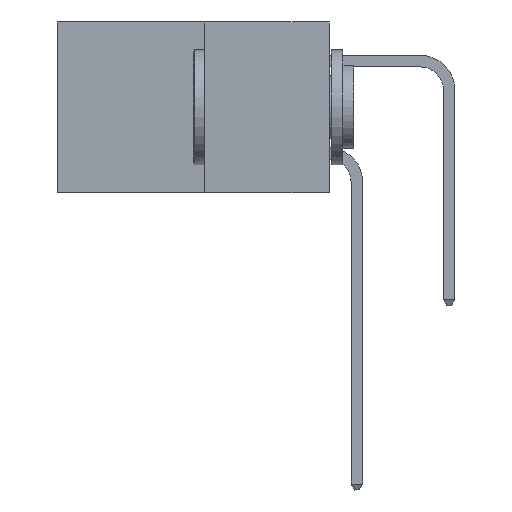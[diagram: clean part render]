
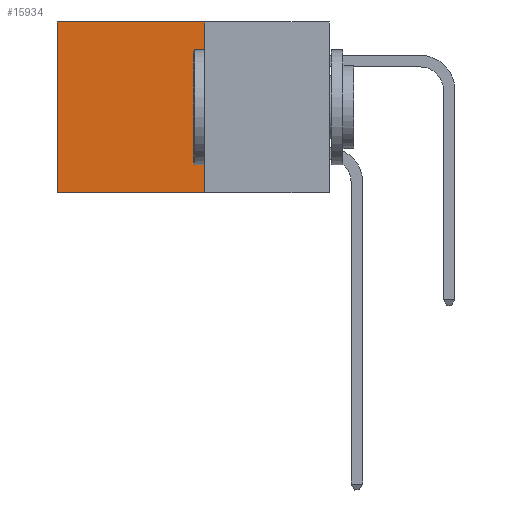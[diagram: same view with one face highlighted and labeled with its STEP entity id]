
A CAD part, left-side view. The second image highlights one B-rep face of the part: STEP entity #15934.
In plain terms, the highlighted planar face has unit normal (-1, 0, 0).
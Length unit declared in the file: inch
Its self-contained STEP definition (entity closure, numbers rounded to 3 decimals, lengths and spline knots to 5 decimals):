
#516 = VECTOR ( 'NONE', #14558, 39.37008 ) ;
#780 = VERTEX_POINT ( 'NONE', #2184 ) ;
#958 = ORIENTED_EDGE ( 'NONE', *, *, #1210, .T. ) ;
#1210 = EDGE_CURVE ( 'NONE', #10271, #9651, #15491, .T. ) ;
#2184 = CARTESIAN_POINT ( 'NONE',  ( 0.277, 0.27, 0. ) ) ;
#3373 = EDGE_CURVE ( 'NONE', #10258, #9651, #12716, .T. ) ;
#3897 = CARTESIAN_POINT ( 'NONE',  ( 0.277, 0.27, 0. ) ) ;
#4128 = CARTESIAN_POINT ( 'NONE',  ( 0.277, 0.59, -0.37 ) ) ;
#5080 = DIRECTION ( 'NONE',  ( 0., 0., -1. ) ) ;
#5265 = CARTESIAN_POINT ( 'NONE',  ( 0.277, 0.27, -0.37 ) ) ;
#5322 = EDGE_LOOP ( 'NONE', ( #958, #7777, #6894, #8088 ) ) ;
#5986 = PLANE ( 'NONE',  #7376 ) ;
#6894 = ORIENTED_EDGE ( 'NONE', *, *, #9607, .F. ) ;
#7307 = DIRECTION ( 'NONE',  ( 0., 0., -1. ) ) ;
#7376 = AXIS2_PLACEMENT_3D ( 'NONE', #11265, #15224, #7307 ) ;
#7544 = LINE ( 'NONE', #13253, #516 ) ;
#7777 = ORIENTED_EDGE ( 'NONE', *, *, #3373, .F. ) ;
#7909 = CARTESIAN_POINT ( 'NONE',  ( 0.277, 0.59, 0. ) ) ;
#8088 = ORIENTED_EDGE ( 'NONE', *, *, #9514, .T. ) ;
#8822 = LINE ( 'NONE', #3897, #15789 ) ;
#9514 = EDGE_CURVE ( 'NONE', #780, #10271, #8822, .T. ) ;
#9607 = EDGE_CURVE ( 'NONE', #780, #10258, #7544, .T. ) ;
#9651 = VERTEX_POINT ( 'NONE', #4128 ) ;
#10088 = CARTESIAN_POINT ( 'NONE',  ( 0.277, 0.59, -0.37 ) ) ;
#10258 = VERTEX_POINT ( 'NONE', #5265 ) ;
#10271 = VERTEX_POINT ( 'NONE', #7909 ) ;
#11265 = CARTESIAN_POINT ( 'NONE',  ( 0.277, 0.27, -0.37 ) ) ;
#12716 = LINE ( 'NONE', #16262, #16561 ) ;
#12839 = FACE_OUTER_BOUND ( 'NONE', #5322, .T. ) ;
#13069 = DIRECTION ( 'NONE',  ( 0., 1., 0. ) ) ;
#13253 = CARTESIAN_POINT ( 'NONE',  ( 0.277, 0.27, -0.37 ) ) ;
#14558 = DIRECTION ( 'NONE',  ( 0., 0., -1. ) ) ;
#14678 = VECTOR ( 'NONE', #5080, 39.37008 ) ;
#15224 = DIRECTION ( 'NONE',  ( 1., 0., 0. ) ) ;
#15485 = DIRECTION ( 'NONE',  ( 0., 1., 0. ) ) ;
#15491 = LINE ( 'NONE', #10088, #14678 ) ;
#15789 = VECTOR ( 'NONE', #13069, 39.37008 ) ;
#15934 = ADVANCED_FACE ( 'NONE', ( #12839 ), #5986, .F. ) ;
#16262 = CARTESIAN_POINT ( 'NONE',  ( 0.277, 0.27, -0.37 ) ) ;
#16561 = VECTOR ( 'NONE', #15485, 39.37008 ) ;
